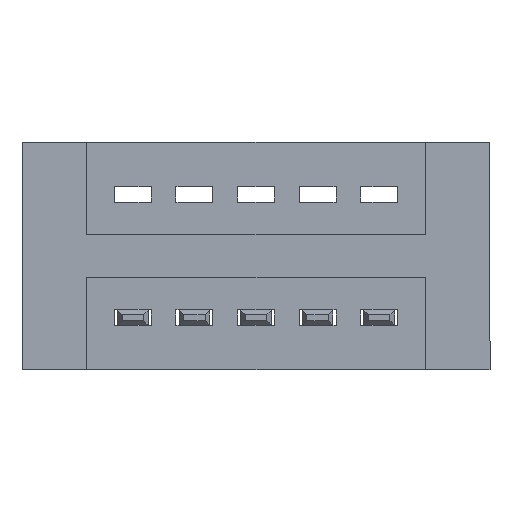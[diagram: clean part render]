
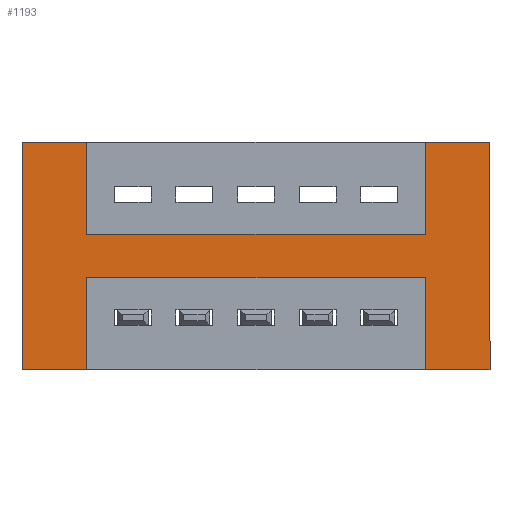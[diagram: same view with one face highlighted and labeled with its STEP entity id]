
A CAD part, front view. The second image highlights one B-rep face of the part: STEP entity #1193.
In plain terms, the highlighted planar face has unit normal (0, -1, 0).
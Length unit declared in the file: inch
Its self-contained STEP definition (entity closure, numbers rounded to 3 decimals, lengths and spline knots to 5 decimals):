
#194 = VECTOR ( 'NONE', #6024, 39.37008 ) ;
#232 = CARTESIAN_POINT ( 'NONE',  ( 0.2875, 0., 0. ) ) ;
#261 = ORIENTED_EDGE ( 'NONE', *, *, #7078, .F. ) ;
#263 = ORIENTED_EDGE ( 'NONE', *, *, #5954, .F. ) ;
#325 = VERTEX_POINT ( 'NONE', #1141 ) ;
#331 = VECTOR ( 'NONE', #691, 39.37008 ) ;
#404 = CARTESIAN_POINT ( 'NONE',  ( 0.9425, 0., -0.37 ) ) ;
#417 = LINE ( 'NONE', #1493, #194 ) ;
#460 = ORIENTED_EDGE ( 'NONE', *, *, #4538, .T. ) ;
#529 = CARTESIAN_POINT ( 'NONE',  ( 1.0475, 0., 0. ) ) ;
#578 = DIRECTION ( 'NONE',  ( 0., 0., -1. ) ) ;
#610 = CARTESIAN_POINT ( 'NONE',  ( 1.0475, 0., 0. ) ) ;
#639 = VERTEX_POINT ( 'NONE', #232 ) ;
#656 = EDGE_CURVE ( 'NONE', #5369, #325, #8133, .T. ) ;
#691 = DIRECTION ( 'NONE',  ( 0., 0., 1. ) ) ;
#1140 = DIRECTION ( 'NONE',  ( 0., 0., 1. ) ) ;
#1141 = CARTESIAN_POINT ( 'NONE',  ( 0.3925, 0., -0.15 ) ) ;
#1193 = ADVANCED_FACE ( 'NONE', ( #4495 ), #2683, .T. ) ;
#1305 = VECTOR ( 'NONE', #7030, 39.37008 ) ;
#1456 = EDGE_CURVE ( 'NONE', #6434, #3704, #3886, .T. ) ;
#1493 = CARTESIAN_POINT ( 'NONE',  ( 0.3925, 0., -0.22 ) ) ;
#1497 = CARTESIAN_POINT ( 'NONE',  ( 0.3925, 0., -0.37 ) ) ;
#1582 = CARTESIAN_POINT ( 'NONE',  ( 0.9425, 0., -0.22 ) ) ;
#1658 = ORIENTED_EDGE ( 'NONE', *, *, #5069, .T. ) ;
#1705 = CARTESIAN_POINT ( 'NONE',  ( 0.3925, 0., 0. ) ) ;
#1765 = VERTEX_POINT ( 'NONE', #1582 ) ;
#1813 = CARTESIAN_POINT ( 'NONE',  ( 0.2875, 0., -0.37 ) ) ;
#1894 = EDGE_CURVE ( 'NONE', #4179, #3686, #3879, .T. ) ;
#2055 = CARTESIAN_POINT ( 'NONE',  ( 1.0475, 0., -0.37 ) ) ;
#2070 = VECTOR ( 'NONE', #4930, 39.37008 ) ;
#2080 = AXIS2_PLACEMENT_3D ( 'NONE', #4126, #4502, #4605 ) ;
#2296 = LINE ( 'NONE', #4194, #3909 ) ;
#2373 = ORIENTED_EDGE ( 'NONE', *, *, #5418, .F. ) ;
#2554 = VERTEX_POINT ( 'NONE', #2055 ) ;
#2567 = CARTESIAN_POINT ( 'NONE',  ( 0.3925, 0., -0.15 ) ) ;
#2683 = PLANE ( 'NONE',  #2080 ) ;
#2689 = VERTEX_POINT ( 'NONE', #610 ) ;
#2802 = VECTOR ( 'NONE', #1140, 39.37008 ) ;
#2810 = CARTESIAN_POINT ( 'NONE',  ( 0., 0., 0. ) ) ;
#2965 = VECTOR ( 'NONE', #7843, 39.37008 ) ;
#3010 = CARTESIAN_POINT ( 'NONE',  ( 0.9425, 0., 0. ) ) ;
#3026 = DIRECTION ( 'NONE',  ( -1., 0., 0. ) ) ;
#3270 = DIRECTION ( 'NONE',  ( 1., 0., 0. ) ) ;
#3418 = VERTEX_POINT ( 'NONE', #4493 ) ;
#3487 = LINE ( 'NONE', #2810, #6489 ) ;
#3498 = DIRECTION ( 'NONE',  ( -1., 0., 0. ) ) ;
#3554 = CARTESIAN_POINT ( 'NONE',  ( 0., 0., -0.37 ) ) ;
#3675 = CARTESIAN_POINT ( 'NONE',  ( 0., 0., 0. ) ) ;
#3686 = VERTEX_POINT ( 'NONE', #1813 ) ;
#3704 = VERTEX_POINT ( 'NONE', #3010 ) ;
#3879 = LINE ( 'NONE', #3554, #5671 ) ;
#3886 = LINE ( 'NONE', #6456, #2070 ) ;
#3890 = EDGE_LOOP ( 'NONE', ( #1658, #261, #7074, #7249, #7865, #2373, #460, #6196, #7874, #4984, #4389, #263 ) ) ;
#3909 = VECTOR ( 'NONE', #3026, 39.37008 ) ;
#4126 = CARTESIAN_POINT ( 'NONE',  ( 0., 0., -0.37 ) ) ;
#4179 = VERTEX_POINT ( 'NONE', #7330 ) ;
#4194 = CARTESIAN_POINT ( 'NONE',  ( 0., 0., -0.37 ) ) ;
#4389 = ORIENTED_EDGE ( 'NONE', *, *, #8246, .F. ) ;
#4422 = CARTESIAN_POINT ( 'NONE',  ( 0.9425, 0., -0.37 ) ) ;
#4485 = LINE ( 'NONE', #529, #331 ) ;
#4493 = CARTESIAN_POINT ( 'NONE',  ( 0.3925, 0., -0.22 ) ) ;
#4495 = FACE_OUTER_BOUND ( 'NONE', #3890, .T. ) ;
#4502 = DIRECTION ( 'NONE',  ( 0., -1., 0. ) ) ;
#4538 = EDGE_CURVE ( 'NONE', #639, #3686, #7565, .T. ) ;
#4605 = DIRECTION ( 'NONE',  ( 0., 0., -1. ) ) ;
#4670 = LINE ( 'NONE', #3675, #2965 ) ;
#4930 = DIRECTION ( 'NONE',  ( 0., 0., 1. ) ) ;
#4984 = ORIENTED_EDGE ( 'NONE', *, *, #7214, .F. ) ;
#5069 = EDGE_CURVE ( 'NONE', #2554, #2689, #4485, .T. ) ;
#5079 = DIRECTION ( 'NONE',  ( 0., 0., -1. ) ) ;
#5095 = LINE ( 'NONE', #2567, #7782 ) ;
#5252 = VECTOR ( 'NONE', #5079, 39.37008 ) ;
#5369 = VERTEX_POINT ( 'NONE', #8296 ) ;
#5418 = EDGE_CURVE ( 'NONE', #639, #5369, #4670, .T. ) ;
#5419 = LINE ( 'NONE', #1497, #6597 ) ;
#5671 = VECTOR ( 'NONE', #3498, 39.37008 ) ;
#5760 = EDGE_CURVE ( 'NONE', #3418, #4179, #5419, .T. ) ;
#5859 = CARTESIAN_POINT ( 'NONE',  ( 0.9425, 0., -0.15 ) ) ;
#5954 = EDGE_CURVE ( 'NONE', #2554, #6884, #2296, .T. ) ;
#6024 = DIRECTION ( 'NONE',  ( -1., 0., 0. ) ) ;
#6196 = ORIENTED_EDGE ( 'NONE', *, *, #1894, .F. ) ;
#6395 = DIRECTION ( 'NONE',  ( 1., 0., 0. ) ) ;
#6434 = VERTEX_POINT ( 'NONE', #5859 ) ;
#6456 = CARTESIAN_POINT ( 'NONE',  ( 0.9425, 0., 0. ) ) ;
#6489 = VECTOR ( 'NONE', #6395, 39.37008 ) ;
#6597 = VECTOR ( 'NONE', #578, 39.37008 ) ;
#6677 = CARTESIAN_POINT ( 'NONE',  ( 0.2875, 0., 0. ) ) ;
#6884 = VERTEX_POINT ( 'NONE', #4422 ) ;
#7030 = DIRECTION ( 'NONE',  ( 0., 0., -1. ) ) ;
#7074 = ORIENTED_EDGE ( 'NONE', *, *, #1456, .F. ) ;
#7078 = EDGE_CURVE ( 'NONE', #3704, #2689, #3487, .T. ) ;
#7214 = EDGE_CURVE ( 'NONE', #1765, #3418, #417, .T. ) ;
#7249 = ORIENTED_EDGE ( 'NONE', *, *, #8206, .F. ) ;
#7330 = CARTESIAN_POINT ( 'NONE',  ( 0.3925, 0., -0.37 ) ) ;
#7565 = LINE ( 'NONE', #6677, #5252 ) ;
#7598 = LINE ( 'NONE', #404, #2802 ) ;
#7782 = VECTOR ( 'NONE', #3270, 39.37008 ) ;
#7843 = DIRECTION ( 'NONE',  ( 1., 0., 0. ) ) ;
#7865 = ORIENTED_EDGE ( 'NONE', *, *, #656, .F. ) ;
#7874 = ORIENTED_EDGE ( 'NONE', *, *, #5760, .F. ) ;
#8133 = LINE ( 'NONE', #1705, #1305 ) ;
#8206 = EDGE_CURVE ( 'NONE', #325, #6434, #5095, .T. ) ;
#8246 = EDGE_CURVE ( 'NONE', #6884, #1765, #7598, .T. ) ;
#8296 = CARTESIAN_POINT ( 'NONE',  ( 0.3925, 0., 0. ) ) ;
